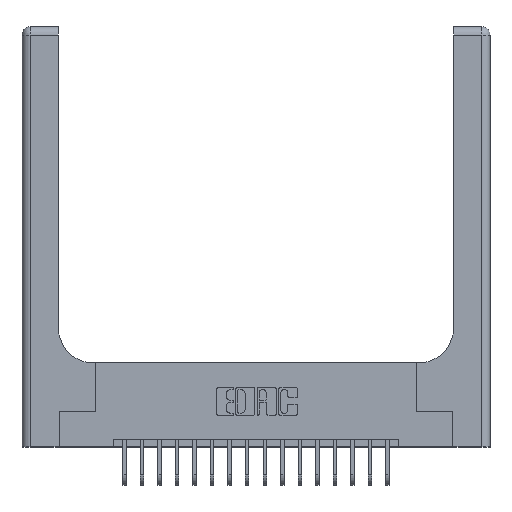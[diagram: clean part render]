
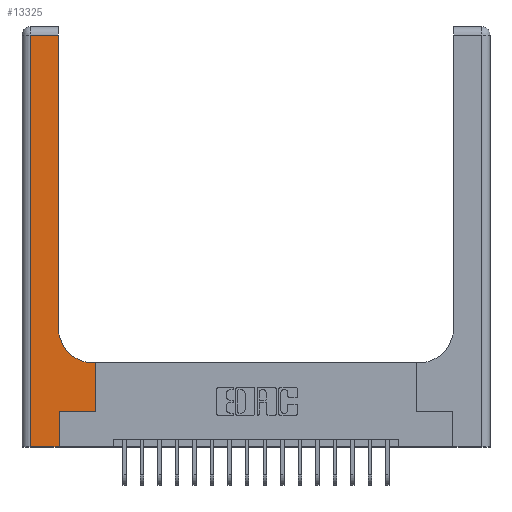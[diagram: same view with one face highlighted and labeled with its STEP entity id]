
A CAD part, top view. The second image highlights one B-rep face of the part: STEP entity #13325.
In plain terms, the highlighted planar face has unit normal (0, 0, 1).
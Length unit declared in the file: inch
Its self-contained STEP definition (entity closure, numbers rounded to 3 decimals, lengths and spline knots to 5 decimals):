
#123 = CARTESIAN_POINT ( 'NONE',  ( 0.265, 0., 0.37 ) ) ;
#411 = VECTOR ( 'NONE', #6635, 39.37008 ) ;
#882 = CARTESIAN_POINT ( 'NONE',  ( 0., 3., 0.37 ) ) ;
#1154 = CARTESIAN_POINT ( 'NONE',  ( 0.06, 0., 0.37 ) ) ;
#1181 = ORIENTED_EDGE ( 'NONE', *, *, #7787, .T. ) ;
#1249 = EDGE_LOOP ( 'NONE', ( #2501, #2557, #6685, #4946, #17424, #1181, #11897, #2037, #10298 ) ) ;
#1390 = CARTESIAN_POINT ( 'NONE',  ( 0.528, 0.6, 0.37 ) ) ;
#1730 = CARTESIAN_POINT ( 'NONE',  ( 0.51, 0.6, 0.37 ) ) ;
#1913 = CARTESIAN_POINT ( 'NONE',  ( 0.06, 3., 0.37 ) ) ;
#2037 = ORIENTED_EDGE ( 'NONE', *, *, #15151, .T. ) ;
#2141 = CARTESIAN_POINT ( 'NONE',  ( 0., 2.94, 0.37 ) ) ;
#2438 = DIRECTION ( 'NONE',  ( 0., 1., 0. ) ) ;
#2501 = ORIENTED_EDGE ( 'NONE', *, *, #9318, .T. ) ;
#2557 = ORIENTED_EDGE ( 'NONE', *, *, #13158, .T. ) ;
#3754 = DIRECTION ( 'NONE',  ( -1., 0., 0. ) ) ;
#3911 = CARTESIAN_POINT ( 'NONE',  ( 0.26, 0.85, 0.37 ) ) ;
#3922 = AXIS2_PLACEMENT_3D ( 'NONE', #17785, #10398, #8969 ) ;
#4001 = EDGE_CURVE ( 'NONE', #16194, #5350, #14096, .T. ) ;
#4069 = CARTESIAN_POINT ( 'NONE',  ( 0.26, 2.94, 0.37 ) ) ;
#4321 = VERTEX_POINT ( 'NONE', #18763 ) ;
#4946 = ORIENTED_EDGE ( 'NONE', *, *, #5675, .T. ) ;
#5214 = CARTESIAN_POINT ( 'NONE',  ( 0.528, 0.25, 0.37 ) ) ;
#5246 = EDGE_CURVE ( 'NONE', #4321, #10989, #12165, .T. ) ;
#5350 = VERTEX_POINT ( 'NONE', #3911 ) ;
#5426 = PLANE ( 'NONE',  #8016 ) ;
#5675 = EDGE_CURVE ( 'NONE', #10989, #10405, #14266, .T. ) ;
#6472 = VECTOR ( 'NONE', #8143, 39.37008 ) ;
#6635 = DIRECTION ( 'NONE',  ( 1., 0., 0. ) ) ;
#6685 = ORIENTED_EDGE ( 'NONE', *, *, #5246, .T. ) ;
#6797 = CARTESIAN_POINT ( 'NONE',  ( 0.26, 3., 0.37 ) ) ;
#6861 = DIRECTION ( 'NONE',  ( 0., 1., 0. ) ) ;
#7638 = DIRECTION ( 'NONE',  ( 0., -1., 0. ) ) ;
#7787 = EDGE_CURVE ( 'NONE', #14214, #8783, #17177, .T. ) ;
#8016 = AXIS2_PLACEMENT_3D ( 'NONE', #882, #8519, #9880 ) ;
#8084 = VECTOR ( 'NONE', #6861, 39.37008 ) ;
#8143 = DIRECTION ( 'NONE',  ( -1., 0., 0. ) ) ;
#8519 = DIRECTION ( 'NONE',  ( 0., 0., -1. ) ) ;
#8593 = VECTOR ( 'NONE', #13365, 39.37008 ) ;
#8661 = VECTOR ( 'NONE', #3754, 39.37008 ) ;
#8783 = VERTEX_POINT ( 'NONE', #15236 ) ;
#8969 = DIRECTION ( 'NONE',  ( 1., 0., 0. ) ) ;
#9318 = EDGE_CURVE ( 'NONE', #5350, #12012, #18698, .T. ) ;
#9880 = DIRECTION ( 'NONE',  ( -1., 0., 0. ) ) ;
#10298 = ORIENTED_EDGE ( 'NONE', *, *, #4001, .T. ) ;
#10398 = DIRECTION ( 'NONE',  ( 0., 0., -1. ) ) ;
#10405 = VERTEX_POINT ( 'NONE', #10939 ) ;
#10570 = LINE ( 'NONE', #2141, #6472 ) ;
#10939 = CARTESIAN_POINT ( 'NONE',  ( 0.265, 0., 0.37 ) ) ;
#10989 = VERTEX_POINT ( 'NONE', #1154 ) ;
#11383 = VERTEX_POINT ( 'NONE', #1390 ) ;
#11762 = EDGE_CURVE ( 'NONE', #10405, #14214, #17754, .T. ) ;
#11897 = ORIENTED_EDGE ( 'NONE', *, *, #16253, .T. ) ;
#12012 = VERTEX_POINT ( 'NONE', #4069 ) ;
#12165 = LINE ( 'NONE', #1913, #16607 ) ;
#12534 = CARTESIAN_POINT ( 'NONE',  ( 0., 0., 0.37 ) ) ;
#12576 = FACE_OUTER_BOUND ( 'NONE', #1249, .T. ) ;
#13158 = EDGE_CURVE ( 'NONE', #12012, #4321, #10570, .T. ) ;
#13325 = ADVANCED_FACE ( 'NONE', ( #12576 ), #5426, .F. ) ;
#13365 = DIRECTION ( 'NONE',  ( 0., 1., 0. ) ) ;
#14096 = CIRCLE ( 'NONE', #3922, 0.25 ) ;
#14214 = VERTEX_POINT ( 'NONE', #15991 ) ;
#14266 = LINE ( 'NONE', #12534, #15049 ) ;
#14340 = CARTESIAN_POINT ( 'NONE',  ( 0.265, 0.25, 0.37 ) ) ;
#15049 = VECTOR ( 'NONE', #15799, 39.37008 ) ;
#15151 = EDGE_CURVE ( 'NONE', #11383, #16194, #17014, .T. ) ;
#15236 = CARTESIAN_POINT ( 'NONE',  ( 0.528, 0.25, 0.37 ) ) ;
#15799 = DIRECTION ( 'NONE',  ( 1., 0., 0. ) ) ;
#15991 = CARTESIAN_POINT ( 'NONE',  ( 0.265, 0.25, 0.37 ) ) ;
#16194 = VERTEX_POINT ( 'NONE', #1730 ) ;
#16253 = EDGE_CURVE ( 'NONE', #8783, #11383, #16919, .T. ) ;
#16607 = VECTOR ( 'NONE', #7638, 39.37008 ) ;
#16919 = LINE ( 'NONE', #5214, #8084 ) ;
#17014 = LINE ( 'NONE', #18572, #8661 ) ;
#17177 = LINE ( 'NONE', #14340, #411 ) ;
#17424 = ORIENTED_EDGE ( 'NONE', *, *, #11762, .T. ) ;
#17754 = LINE ( 'NONE', #123, #8593 ) ;
#17785 = CARTESIAN_POINT ( 'NONE',  ( 0.51, 0.85, 0.37 ) ) ;
#18531 = VECTOR ( 'NONE', #2438, 39.37008 ) ;
#18572 = CARTESIAN_POINT ( 'NONE',  ( 0.26, 0.6, 0.37 ) ) ;
#18698 = LINE ( 'NONE', #6797, #18531 ) ;
#18763 = CARTESIAN_POINT ( 'NONE',  ( 0.06, 2.94, 0.37 ) ) ;
